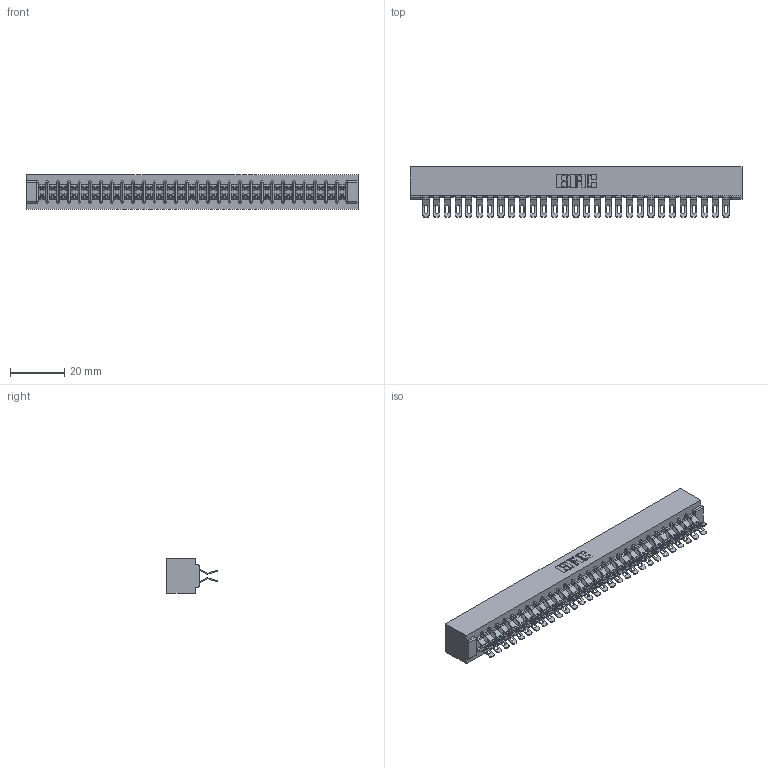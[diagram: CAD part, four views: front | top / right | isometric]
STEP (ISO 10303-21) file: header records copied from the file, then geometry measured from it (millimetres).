
FILE_DESCRIPTION (( 'STEP AP203' ), '1' );
FILE_NAME ('357-058-555-201.STEP', '2018-08-12T14:17:49', ( '' ), ( '' ), 'SwSTEP 2.0', 'SolidWorks 2016', '' );
FILE_SCHEMA (( 'CONFIG_CONTROL_DESIGN' ));
Length unit declared in the file: inch
Products named in the file (3): 307 Part_No Mounting Lugs; 307-290-001_555; 357-058-555-201
Assembly tree (59 placements, depth 2):
  357-058-555-201
    307 Part_No Mounting Lugs
    307-290-001_555  x58
Bounding box: 122.78 x 18.75 x 12.7 mm (x, y, z)
Volume: 13684.8 mm3; surface area: 17755.8 mm2
Topology: 59 solids, 59 shells, 3678 faces, 10797 edges, 7038 vertices
Faces by surface type: plane 2038, cylinder 1580, sphere 60
Entity records: 27651 total; most frequent: CARTESIAN_POINT 4529, ORIENTED_EDGE 4488, DIRECTION 4448, EDGE_CURVE 2244, VECTOR 1706, LINE 1706, VERTEX_POINT 1452, AXIS2_PLACEMENT_3D 1371
